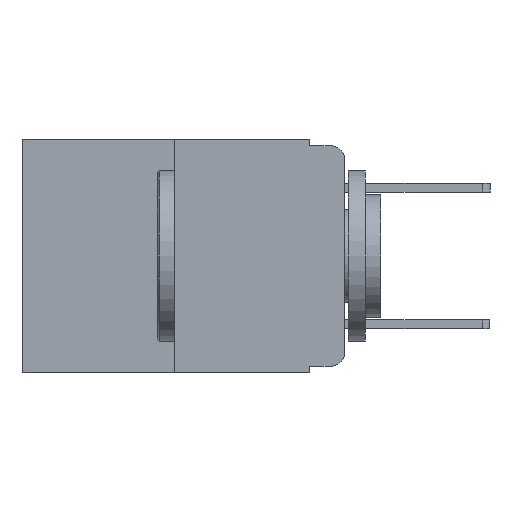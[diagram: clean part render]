
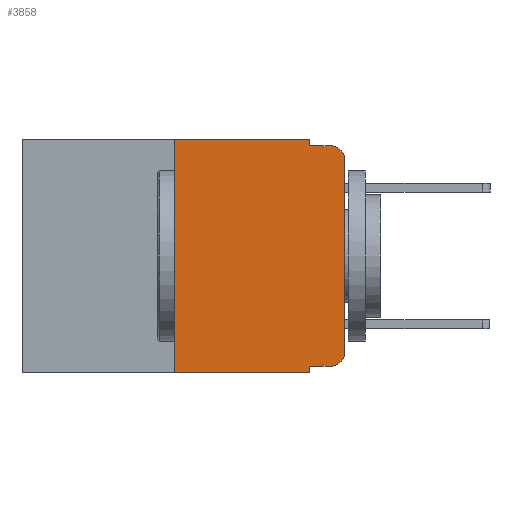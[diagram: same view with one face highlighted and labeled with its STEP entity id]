
A CAD part, left-side view. The second image highlights one B-rep face of the part: STEP entity #3858.
In plain terms, the highlighted planar face has unit normal (-1, 0, 0).
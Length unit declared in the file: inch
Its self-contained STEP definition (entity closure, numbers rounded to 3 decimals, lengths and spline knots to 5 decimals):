
#187 = ORIENTED_EDGE ( 'NONE', *, *, #6350, .F. ) ;
#890 = EDGE_CURVE ( 'NONE', #2952, #14394, #18608, .T. ) ;
#915 = VERTEX_POINT ( 'NONE', #17667 ) ;
#1172 = CARTESIAN_POINT ( 'NONE',  ( 0., 0.25, 0. ) ) ;
#1536 = VERTEX_POINT ( 'NONE', #11671 ) ;
#1623 = CARTESIAN_POINT ( 'NONE',  ( 0., 0.051, 0. ) ) ;
#1636 = DIRECTION ( 'NONE',  ( 0., -1., 0. ) ) ;
#1674 = DIRECTION ( 'NONE',  ( 0., -1., 0. ) ) ;
#2087 = VERTEX_POINT ( 'NONE', #15997 ) ;
#2149 = VECTOR ( 'NONE', #17635, 39.37008 ) ;
#2300 = CARTESIAN_POINT ( 'NONE',  ( 0., 0., -0.313 ) ) ;
#2359 = VECTOR ( 'NONE', #1674, 39.37008 ) ;
#2952 = VERTEX_POINT ( 'NONE', #7653 ) ;
#3155 = PLANE ( 'NONE',  #9324 ) ;
#3289 = DIRECTION ( 'NONE',  ( 0., 0., -1. ) ) ;
#3406 = CARTESIAN_POINT ( 'NONE',  ( 0., 0.02, -0.333 ) ) ;
#3667 = LINE ( 'NONE', #6432, #11512 ) ;
#3817 = DIRECTION ( 'NONE',  ( -1., 0., 0. ) ) ;
#3858 = ADVANCED_FACE ( 'NONE', ( #5667 ), #3155, .F. ) ;
#3891 = DIRECTION ( 'NONE',  ( -1., 0., 0. ) ) ;
#3923 = EDGE_CURVE ( 'NONE', #14394, #2087, #3667, .T. ) ;
#4043 = VERTEX_POINT ( 'NONE', #11342 ) ;
#4322 = EDGE_CURVE ( 'NONE', #15481, #4043, #4629, .T. ) ;
#4366 = VERTEX_POINT ( 'NONE', #1172 ) ;
#4629 = LINE ( 'NONE', #12109, #11968 ) ;
#4757 = DIRECTION ( 'NONE',  ( 1., 0., 0. ) ) ;
#5419 = CARTESIAN_POINT ( 'NONE',  ( 0., 0.25, 0. ) ) ;
#5441 = VECTOR ( 'NONE', #3289, 39.37008 ) ;
#5667 = FACE_OUTER_BOUND ( 'NONE', #15297, .T. ) ;
#6011 = VECTOR ( 'NONE', #18381, 39.37008 ) ;
#6350 = EDGE_CURVE ( 'NONE', #4366, #2952, #12985, .T. ) ;
#6432 = CARTESIAN_POINT ( 'NONE',  ( 0., 0.051, -0.01 ) ) ;
#6536 = CARTESIAN_POINT ( 'NONE',  ( 0., 0.051, -0.333 ) ) ;
#6604 = LINE ( 'NONE', #6536, #2359 ) ;
#6767 = ORIENTED_EDGE ( 'NONE', *, *, #4322, .T. ) ;
#6933 = CARTESIAN_POINT ( 'NONE',  ( 0., 0.473, -0.343 ) ) ;
#7399 = EDGE_CURVE ( 'NONE', #1536, #4366, #11071, .T. ) ;
#7527 = VERTEX_POINT ( 'NONE', #13508 ) ;
#7619 = ORIENTED_EDGE ( 'NONE', *, *, #17561, .T. ) ;
#7653 = CARTESIAN_POINT ( 'NONE',  ( 0., 0.051, 0. ) ) ;
#7882 = ORIENTED_EDGE ( 'NONE', *, *, #10543, .F. ) ;
#8498 = VERTEX_POINT ( 'NONE', #3406 ) ;
#9178 = DIRECTION ( 'NONE',  ( 0., -1., 0. ) ) ;
#9324 = AXIS2_PLACEMENT_3D ( 'NONE', #11020, #4757, #15525 ) ;
#9512 = ORIENTED_EDGE ( 'NONE', *, *, #14568, .T. ) ;
#9633 = LINE ( 'NONE', #1623, #5441 ) ;
#9690 = EDGE_CURVE ( 'NONE', #1536, #915, #18516, .T. ) ;
#10199 = ORIENTED_EDGE ( 'NONE', *, *, #7399, .F. ) ;
#10425 = ORIENTED_EDGE ( 'NONE', *, *, #9690, .T. ) ;
#10428 = AXIS2_PLACEMENT_3D ( 'NONE', #13125, #3817, #14650 ) ;
#10543 = EDGE_CURVE ( 'NONE', #7527, #915, #9633, .T. ) ;
#10603 = VECTOR ( 'NONE', #13118, 39.37008 ) ;
#10788 = CARTESIAN_POINT ( 'NONE',  ( 0., 0.051, -0.01 ) ) ;
#11020 = CARTESIAN_POINT ( 'NONE',  ( 0., 0.473, 0. ) ) ;
#11071 = LINE ( 'NONE', #5419, #2149 ) ;
#11342 = CARTESIAN_POINT ( 'NONE',  ( 0., 0., -0.03 ) ) ;
#11512 = VECTOR ( 'NONE', #1636, 39.37008 ) ;
#11536 = CARTESIAN_POINT ( 'NONE',  ( 0., 0.051, 0. ) ) ;
#11661 = EDGE_CURVE ( 'NONE', #4043, #2087, #19475, .T. ) ;
#11671 = CARTESIAN_POINT ( 'NONE',  ( 0., 0.25, -0.343 ) ) ;
#11968 = VECTOR ( 'NONE', #19493, 39.37008 ) ;
#12109 = CARTESIAN_POINT ( 'NONE',  ( 0., 0., 0. ) ) ;
#12985 = LINE ( 'NONE', #18184, #13449 ) ;
#13118 = DIRECTION ( 'NONE',  ( 0., -1., 0. ) ) ;
#13125 = CARTESIAN_POINT ( 'NONE',  ( 0., 0.02, -0.313 ) ) ;
#13196 = CARTESIAN_POINT ( 'NONE',  ( 0., 0.02, -0.03 ) ) ;
#13449 = VECTOR ( 'NONE', #9178, 39.37008 ) ;
#13508 = CARTESIAN_POINT ( 'NONE',  ( 0., 0.051, -0.333 ) ) ;
#14330 = ORIENTED_EDGE ( 'NONE', *, *, #3923, .F. ) ;
#14394 = VERTEX_POINT ( 'NONE', #10788 ) ;
#14568 = EDGE_CURVE ( 'NONE', #7527, #8498, #6604, .T. ) ;
#14650 = DIRECTION ( 'NONE',  ( 0., 0., -1. ) ) ;
#14721 = DIRECTION ( 'NONE',  ( 0., 0., -1. ) ) ;
#15297 = EDGE_LOOP ( 'NONE', ( #6767, #19170, #14330, #17212, #187, #10199, #10425, #7882, #9512, #7619 ) ) ;
#15481 = VERTEX_POINT ( 'NONE', #2300 ) ;
#15525 = DIRECTION ( 'NONE',  ( 0., 0., -1. ) ) ;
#15650 = CIRCLE ( 'NONE', #10428, 0.02 ) ;
#15997 = CARTESIAN_POINT ( 'NONE',  ( 0., 0.02, -0.01 ) ) ;
#17212 = ORIENTED_EDGE ( 'NONE', *, *, #890, .F. ) ;
#17561 = EDGE_CURVE ( 'NONE', #8498, #15481, #15650, .T. ) ;
#17635 = DIRECTION ( 'NONE',  ( 0., 0., 1. ) ) ;
#17667 = CARTESIAN_POINT ( 'NONE',  ( 0., 0.051, -0.343 ) ) ;
#18184 = CARTESIAN_POINT ( 'NONE',  ( 0., 0.473, 0. ) ) ;
#18381 = DIRECTION ( 'NONE',  ( 0., 0., -1. ) ) ;
#18516 = LINE ( 'NONE', #6933, #10603 ) ;
#18608 = LINE ( 'NONE', #11536, #6011 ) ;
#18961 = AXIS2_PLACEMENT_3D ( 'NONE', #13196, #3891, #14721 ) ;
#19170 = ORIENTED_EDGE ( 'NONE', *, *, #11661, .T. ) ;
#19475 = CIRCLE ( 'NONE', #18961, 0.02 ) ;
#19493 = DIRECTION ( 'NONE',  ( 0., 0., 1. ) ) ;
